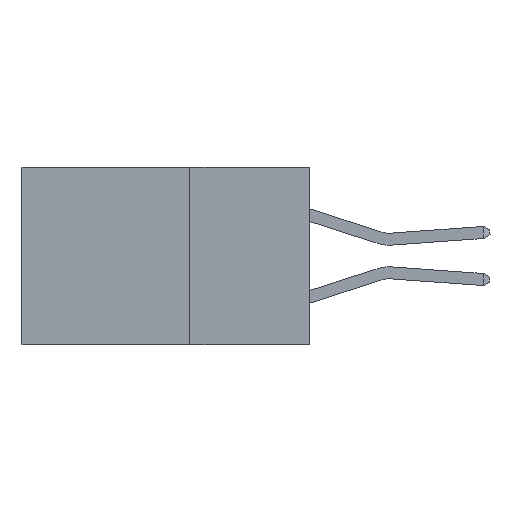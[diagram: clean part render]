
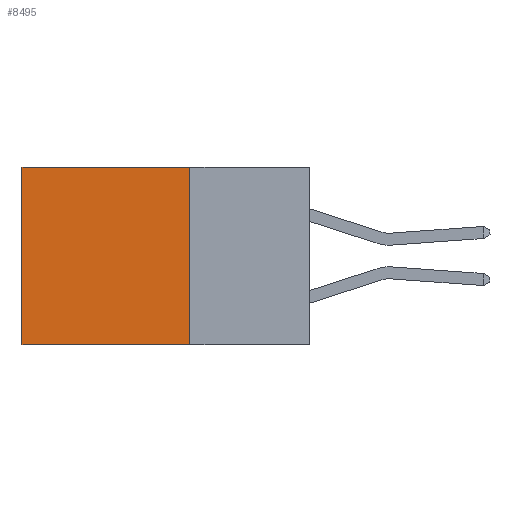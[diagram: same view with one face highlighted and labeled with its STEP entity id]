
A CAD part, left-side view. The second image highlights one B-rep face of the part: STEP entity #8495.
In plain terms, the highlighted planar face has unit normal (-1, 0, 0).
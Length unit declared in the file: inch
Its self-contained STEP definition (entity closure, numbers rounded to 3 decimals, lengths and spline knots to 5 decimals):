
#511 = LINE ( 'NONE', #576, #7632 ) ;
#576 = CARTESIAN_POINT ( 'NONE',  ( 0.298, 0.25, 0. ) ) ;
#747 = CARTESIAN_POINT ( 'NONE',  ( 0.298, 0.25, 0. ) ) ;
#1064 = ORIENTED_EDGE ( 'NONE', *, *, #5598, .T. ) ;
#1077 = CARTESIAN_POINT ( 'NONE',  ( 0.298, 0.6, -0.37 ) ) ;
#1419 = AXIS2_PLACEMENT_3D ( 'NONE', #747, #7251, #1664 ) ;
#1664 = DIRECTION ( 'NONE',  ( 0., 0., -1. ) ) ;
#2264 = ORIENTED_EDGE ( 'NONE', *, *, #10846, .F. ) ;
#2705 = LINE ( 'NONE', #5723, #10113 ) ;
#2877 = EDGE_LOOP ( 'NONE', ( #1064, #10868, #2264, #5285 ) ) ;
#3321 = DIRECTION ( 'NONE',  ( 0., 0., -1. ) ) ;
#3662 = LINE ( 'NONE', #9192, #5542 ) ;
#4256 = CARTESIAN_POINT ( 'NONE',  ( 0.298, 0.6, 0. ) ) ;
#4562 = CARTESIAN_POINT ( 'NONE',  ( 0.298, 0.25, 0. ) ) ;
#4724 = EDGE_CURVE ( 'NONE', #8063, #9868, #2705, .T. ) ;
#5125 = DIRECTION ( 'NONE',  ( 0., 1., 0. ) ) ;
#5285 = ORIENTED_EDGE ( 'NONE', *, *, #11934, .T. ) ;
#5542 = VECTOR ( 'NONE', #9156, 39.37008 ) ;
#5598 = EDGE_CURVE ( 'NONE', #9819, #9868, #7654, .T. ) ;
#5723 = CARTESIAN_POINT ( 'NONE',  ( 0.298, 0.25, -0.37 ) ) ;
#6424 = CARTESIAN_POINT ( 'NONE',  ( 0.298, 0.6, 0. ) ) ;
#6850 = FACE_OUTER_BOUND ( 'NONE', #2877, .T. ) ;
#7031 = CARTESIAN_POINT ( 'NONE',  ( 0.298, 0.25, -0.37 ) ) ;
#7075 = VECTOR ( 'NONE', #3321, 39.37008 ) ;
#7251 = DIRECTION ( 'NONE',  ( 1., 0., 0. ) ) ;
#7632 = VECTOR ( 'NONE', #11682, 39.37008 ) ;
#7654 = LINE ( 'NONE', #4256, #7075 ) ;
#8063 = VERTEX_POINT ( 'NONE', #7031 ) ;
#8495 = ADVANCED_FACE ( 'NONE', ( #6850 ), #11860, .F. ) ;
#9156 = DIRECTION ( 'NONE',  ( 0., 1., 0. ) ) ;
#9192 = CARTESIAN_POINT ( 'NONE',  ( 0.298, 0.25, 0. ) ) ;
#9819 = VERTEX_POINT ( 'NONE', #6424 ) ;
#9868 = VERTEX_POINT ( 'NONE', #1077 ) ;
#10113 = VECTOR ( 'NONE', #5125, 39.37008 ) ;
#10846 = EDGE_CURVE ( 'NONE', #11940, #8063, #511, .T. ) ;
#10868 = ORIENTED_EDGE ( 'NONE', *, *, #4724, .F. ) ;
#11682 = DIRECTION ( 'NONE',  ( 0., 0., -1. ) ) ;
#11860 = PLANE ( 'NONE',  #1419 ) ;
#11934 = EDGE_CURVE ( 'NONE', #11940, #9819, #3662, .T. ) ;
#11940 = VERTEX_POINT ( 'NONE', #4562 ) ;
